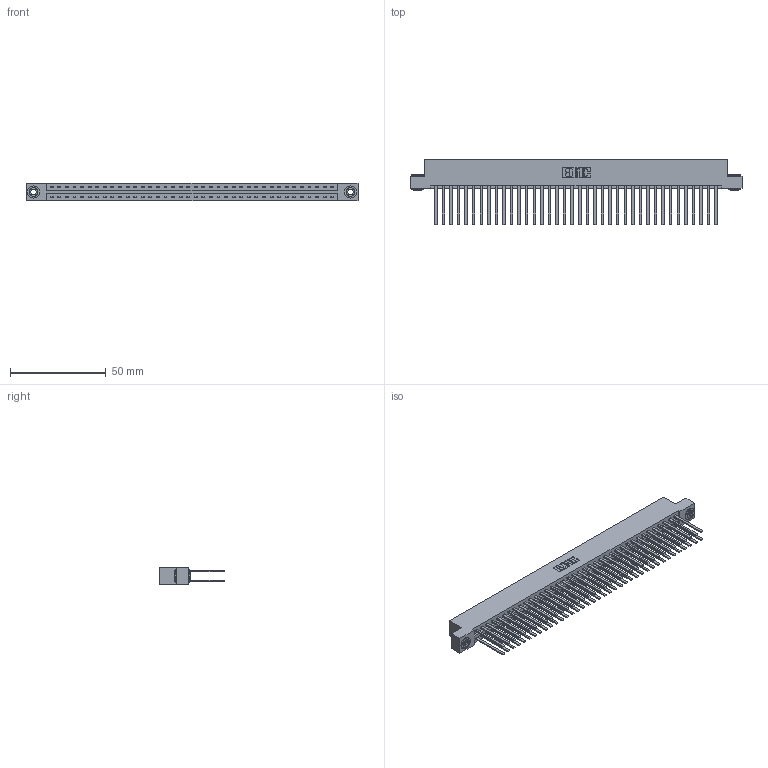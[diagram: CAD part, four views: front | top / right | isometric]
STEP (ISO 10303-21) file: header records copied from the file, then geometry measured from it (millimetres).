
FILE_DESCRIPTION (( 'STEP AP203' ), '1' );
FILE_NAME ('337-076-544-203.STEP', '2019-10-10T10:46:46', ( '' ), ( '' ), 'SwSTEP 2.0', 'SolidWorks 2016', '' );
FILE_SCHEMA (( 'CONFIG_CONTROL_DESIGN' ));
Length unit declared in the file: inch
Products named in the file (4): 345-292-001_345-293-144; 337 Part_Flush Mounting Lugs - 0.156 Dia-TH; 337-076-544-203; 345-250-002_345-250-002-102
Assembly tree (79 placements, depth 2):
  337-076-544-203
    337 Part_Flush Mounting Lugs - 0.156 Dia-TH
    345-292-001_345-293-144  x76
    345-250-002_345-250-002-102  x2
Bounding box: 173.58 x 34.3 x 9.4 mm (x, y, z)
Volume: 19325.1 mm3; surface area: 25513 mm2
Topology: 79 solids, 79 shells, 3800 faces, 11255 edges, 7398 vertices
Faces by surface type: plane 2664, cylinder 1128, cone 8
Entity records: 30446 total; most frequent: CARTESIAN_POINT 5105, ORIENTED_EDGE 5034, DIRECTION 4379, EDGE_CURVE 2517, VECTOR 2369, LINE 2369, VERTEX_POINT 1674, AXIS2_PLACEMENT_3D 1005
